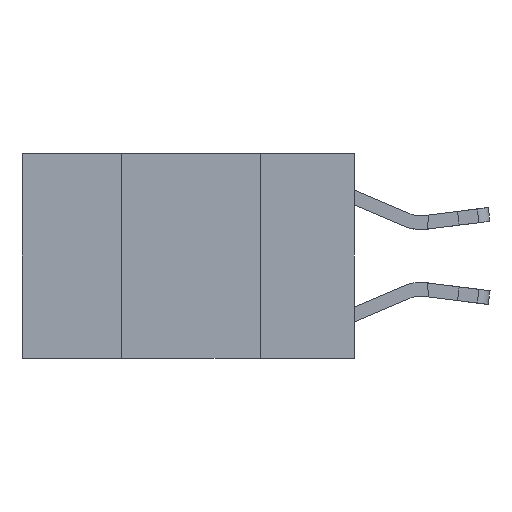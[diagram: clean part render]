
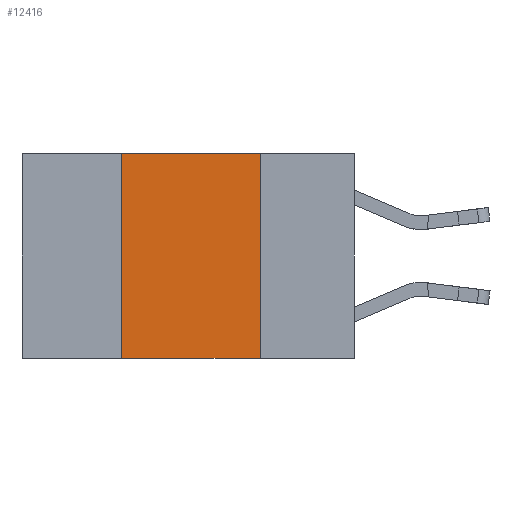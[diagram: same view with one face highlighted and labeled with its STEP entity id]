
A CAD part, left-side view. The second image highlights one B-rep face of the part: STEP entity #12416.
In plain terms, the highlighted planar face has unit normal (-1, 0, 0).
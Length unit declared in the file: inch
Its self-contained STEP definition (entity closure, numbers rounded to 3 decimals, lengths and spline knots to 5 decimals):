
#176 = VECTOR ( 'NONE', #9475, 39.37008 ) ;
#268 = CARTESIAN_POINT ( 'NONE',  ( 0., 0.42, 0. ) ) ;
#306 = LINE ( 'NONE', #13892, #18664 ) ;
#596 = FACE_OUTER_BOUND ( 'NONE', #14008, .T. ) ;
#798 = DIRECTION ( 'NONE',  ( 0., -1., 0. ) ) ;
#1288 = PLANE ( 'NONE',  #16751 ) ;
#4359 = DIRECTION ( 'NONE',  ( 0., 0., -1. ) ) ;
#5833 = LINE ( 'NONE', #6836, #16737 ) ;
#5971 = ORIENTED_EDGE ( 'NONE', *, *, #11650, .F. ) ;
#6463 = ORIENTED_EDGE ( 'NONE', *, *, #13909, .F. ) ;
#6836 = CARTESIAN_POINT ( 'NONE',  ( 0., 0.6, 0. ) ) ;
#7270 = CARTESIAN_POINT ( 'NONE',  ( 0., 0.17, 0. ) ) ;
#8232 = LINE ( 'NONE', #13926, #176 ) ;
#8455 = VERTEX_POINT ( 'NONE', #7270 ) ;
#9475 = DIRECTION ( 'NONE',  ( 0., 0., -1. ) ) ;
#9893 = VERTEX_POINT ( 'NONE', #268 ) ;
#10850 = CARTESIAN_POINT ( 'NONE',  ( 0., 0.6, -0.37 ) ) ;
#11500 = EDGE_CURVE ( 'NONE', #8455, #17618, #8232, .T. ) ;
#11650 = EDGE_CURVE ( 'NONE', #9893, #8455, #5833, .T. ) ;
#11820 = CARTESIAN_POINT ( 'NONE',  ( 0., 0.6, 0. ) ) ;
#12416 = ADVANCED_FACE ( 'NONE', ( #596 ), #1288, .F. ) ;
#12675 = LINE ( 'NONE', #10850, #16569 ) ;
#12795 = ORIENTED_EDGE ( 'NONE', *, *, #15690, .T. ) ;
#13312 = DIRECTION ( 'NONE',  ( 1., 0., 0. ) ) ;
#13892 = CARTESIAN_POINT ( 'NONE',  ( 0., 0.42, 0. ) ) ;
#13909 = EDGE_CURVE ( 'NONE', #18727, #9893, #306, .T. ) ;
#13926 = CARTESIAN_POINT ( 'NONE',  ( 0., 0.17, 0. ) ) ;
#14008 = EDGE_LOOP ( 'NONE', ( #14791, #5971, #6463, #12795 ) ) ;
#14791 = ORIENTED_EDGE ( 'NONE', *, *, #11500, .F. ) ;
#15690 = EDGE_CURVE ( 'NONE', #18727, #17618, #12675, .T. ) ;
#16569 = VECTOR ( 'NONE', #16708, 39.37008 ) ;
#16708 = DIRECTION ( 'NONE',  ( 0., -1., 0. ) ) ;
#16737 = VECTOR ( 'NONE', #798, 39.37008 ) ;
#16751 = AXIS2_PLACEMENT_3D ( 'NONE', #11820, #13312, #4359 ) ;
#16945 = CARTESIAN_POINT ( 'NONE',  ( 0., 0.42, -0.37 ) ) ;
#17618 = VERTEX_POINT ( 'NONE', #18601 ) ;
#18276 = DIRECTION ( 'NONE',  ( 0., 0., 1. ) ) ;
#18601 = CARTESIAN_POINT ( 'NONE',  ( 0., 0.17, -0.37 ) ) ;
#18664 = VECTOR ( 'NONE', #18276, 39.37008 ) ;
#18727 = VERTEX_POINT ( 'NONE', #16945 ) ;
